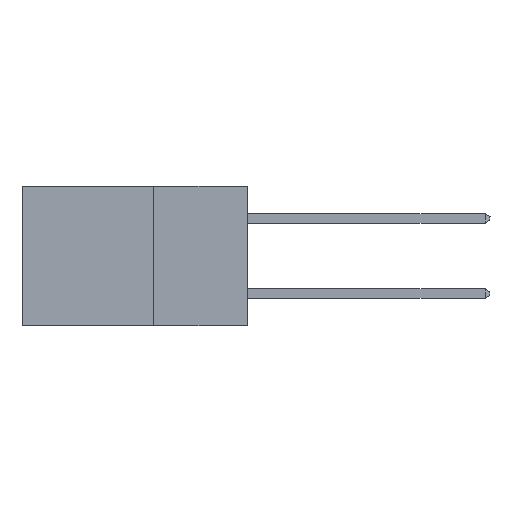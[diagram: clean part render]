
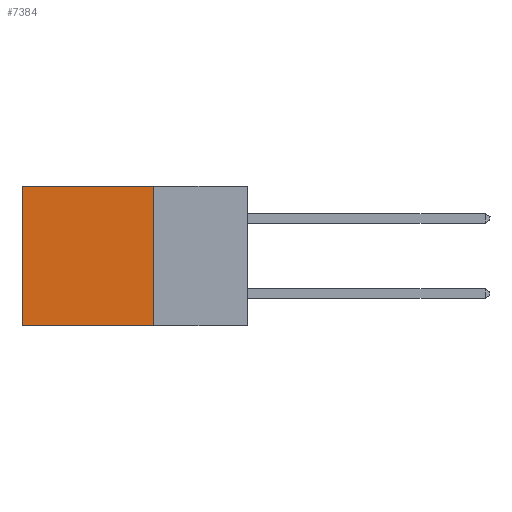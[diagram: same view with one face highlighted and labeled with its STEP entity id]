
A CAD part, left-side view. The second image highlights one B-rep face of the part: STEP entity #7384.
In plain terms, the highlighted planar face has unit normal (-1, 0, 0).
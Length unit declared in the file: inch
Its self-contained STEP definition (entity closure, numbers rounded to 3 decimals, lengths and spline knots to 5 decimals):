
#152 = VERTEX_POINT ( 'NONE', #1024 ) ;
#1024 = CARTESIAN_POINT ( 'NONE',  ( 0.298, 0.25, 0. ) ) ;
#1123 = VECTOR ( 'NONE', #6115, 39.37008 ) ;
#1534 = VECTOR ( 'NONE', #11182, 39.37008 ) ;
#1751 = DIRECTION ( 'NONE',  ( 0., 0., -1. ) ) ;
#2017 = DIRECTION ( 'NONE',  ( 0., 0., -1. ) ) ;
#2142 = VERTEX_POINT ( 'NONE', #16561 ) ;
#2467 = EDGE_LOOP ( 'NONE', ( #18058, #3125, #4816, #15316 ) ) ;
#3125 = ORIENTED_EDGE ( 'NONE', *, *, #10008, .F. ) ;
#4470 = DIRECTION ( 'NONE',  ( 0., 1., 0. ) ) ;
#4645 = LINE ( 'NONE', #12986, #16617 ) ;
#4757 = PLANE ( 'NONE',  #7606 ) ;
#4816 = ORIENTED_EDGE ( 'NONE', *, *, #16408, .F. ) ;
#5067 = LINE ( 'NONE', #16157, #7933 ) ;
#5536 = VERTEX_POINT ( 'NONE', #11397 ) ;
#6115 = DIRECTION ( 'NONE',  ( 0., 1., 0. ) ) ;
#7042 = CARTESIAN_POINT ( 'NONE',  ( 0.298, 0.6, 0. ) ) ;
#7384 = ADVANCED_FACE ( 'NONE', ( #7575 ), #4757, .F. ) ;
#7528 = CARTESIAN_POINT ( 'NONE',  ( 0.298, 0.25, -0.37 ) ) ;
#7575 = FACE_OUTER_BOUND ( 'NONE', #2467, .T. ) ;
#7606 = AXIS2_PLACEMENT_3D ( 'NONE', #13090, #10386, #1751 ) ;
#7933 = VECTOR ( 'NONE', #2017, 39.37008 ) ;
#8961 = EDGE_CURVE ( 'NONE', #152, #2142, #4645, .T. ) ;
#10008 = EDGE_CURVE ( 'NONE', #5536, #14419, #16593, .T. ) ;
#10386 = DIRECTION ( 'NONE',  ( 1., 0., 0. ) ) ;
#11182 = DIRECTION ( 'NONE',  ( 0., 0., -1. ) ) ;
#11319 = EDGE_CURVE ( 'NONE', #2142, #14419, #12784, .T. ) ;
#11397 = CARTESIAN_POINT ( 'NONE',  ( 0.298, 0.25, -0.37 ) ) ;
#12784 = LINE ( 'NONE', #7042, #1534 ) ;
#12986 = CARTESIAN_POINT ( 'NONE',  ( 0.298, 0.25, 0. ) ) ;
#13090 = CARTESIAN_POINT ( 'NONE',  ( 0.298, 0.25, 0. ) ) ;
#14419 = VERTEX_POINT ( 'NONE', #14581 ) ;
#14581 = CARTESIAN_POINT ( 'NONE',  ( 0.298, 0.6, -0.37 ) ) ;
#15316 = ORIENTED_EDGE ( 'NONE', *, *, #8961, .T. ) ;
#16157 = CARTESIAN_POINT ( 'NONE',  ( 0.298, 0.25, 0. ) ) ;
#16408 = EDGE_CURVE ( 'NONE', #152, #5536, #5067, .T. ) ;
#16561 = CARTESIAN_POINT ( 'NONE',  ( 0.298, 0.6, 0. ) ) ;
#16593 = LINE ( 'NONE', #7528, #1123 ) ;
#16617 = VECTOR ( 'NONE', #4470, 39.37008 ) ;
#18058 = ORIENTED_EDGE ( 'NONE', *, *, #11319, .T. ) ;
